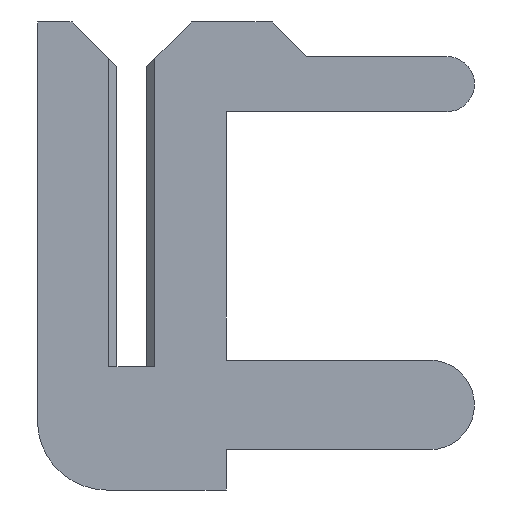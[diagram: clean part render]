
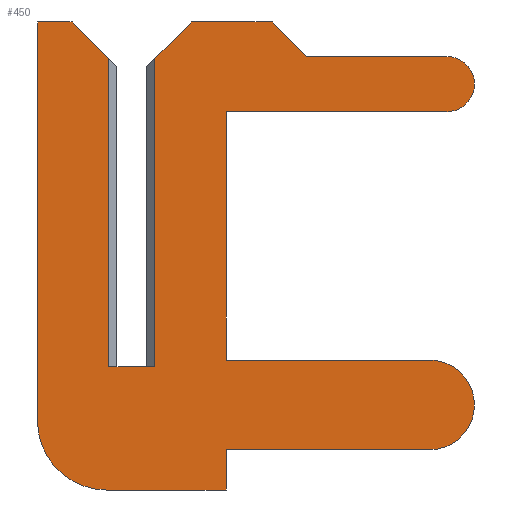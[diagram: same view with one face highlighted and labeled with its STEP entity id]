
A CAD part, left-side view. The second image highlights one B-rep face of the part: STEP entity #450.
In plain terms, the highlighted planar face has unit normal (-1, 0, 0).
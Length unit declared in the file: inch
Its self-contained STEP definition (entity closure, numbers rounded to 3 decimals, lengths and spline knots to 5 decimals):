
#2 = EDGE_CURVE ( 'NONE', #1318, #54, #545, .T. ) ;
#14 = VERTEX_POINT ( 'NONE', #548 ) ;
#23 = DIRECTION ( 'NONE',  ( 0., 0., 1. ) ) ;
#27 = DIRECTION ( 'NONE',  ( 0., -1., 0. ) ) ;
#28 = CARTESIAN_POINT ( 'NONE',  ( -0.01, -0.041, -0.0535 ) ) ;
#37 = ORIENTED_EDGE ( 'NONE', *, *, #387, .F. ) ;
#54 = VERTEX_POINT ( 'NONE', #367 ) ;
#55 = EDGE_CURVE ( 'NONE', #54, #898, #498, .T. ) ;
#56 = CARTESIAN_POINT ( 'NONE',  ( -0.01, 0.01, -0.0235 ) ) ;
#67 = ORIENTED_EDGE ( 'NONE', *, *, #483, .F. ) ;
#74 = EDGE_CURVE ( 'NONE', #751, #1318, #512, .T. ) ;
#81 = CARTESIAN_POINT ( 'NONE',  ( -0.01, -0.041, 0.111 ) ) ;
#88 = EDGE_CURVE ( 'NONE', #524, #998, #677, .T. ) ;
#91 = VECTOR ( 'NONE', #1185, 39.37008 ) ;
#104 = LINE ( 'NONE', #488, #641 ) ;
#136 = VERTEX_POINT ( 'NONE', #81 ) ;
#157 = CARTESIAN_POINT ( 'NONE',  ( -0.01, -0.041, -0.036 ) ) ;
#161 = VECTOR ( 'NONE', #27, 39.37008 ) ;
#166 = DIRECTION ( 'NONE',  ( 0., 0., -1. ) ) ;
#176 = ORIENTED_EDGE ( 'NONE', *, *, #1001, .F. ) ;
#197 = LINE ( 'NONE', #1285, #1102 ) ;
#202 = DIRECTION ( 'NONE',  ( 0., -1., 0. ) ) ;
#209 = CARTESIAN_POINT ( 'NONE',  ( -0.01, -0.01, 0. ) ) ;
#228 = DIRECTION ( 'NONE',  ( 1., 0., 0. ) ) ;
#237 = VERTEX_POINT ( 'NONE', #815 ) ;
#244 = VECTOR ( 'NONE', #202, 39.37008 ) ;
#256 = VERTEX_POINT ( 'NONE', #1148 ) ;
#277 = DIRECTION ( 'NONE',  ( 0., 1., 0. ) ) ;
#278 = CARTESIAN_POINT ( 'NONE',  ( -0.01, -0.061, 0.15 ) ) ;
#291 = EDGE_LOOP ( 'NONE', ( #753, #1279, #332, #1259, #1330, #462, #1212, #788, #603, #879, #866, #913, #1183, #1315, #67, #1342, #808, #37, #176 ) ) ;
#296 = CARTESIAN_POINT ( 'NONE',  ( -0.01, 0.041, 0.15 ) ) ;
#312 = DIRECTION ( 'NONE',  ( 0., -1., 0. ) ) ;
#331 = DIRECTION ( 'NONE',  ( 0., -0.707, 0.707 ) ) ;
#332 = ORIENTED_EDGE ( 'NONE', *, *, #401, .F. ) ;
#340 = DIRECTION ( 'NONE',  ( 0., -0.707, -0.707 ) ) ;
#341 = DIRECTION ( 'NONE',  ( 0., 0., -1. ) ) ;
#350 = EDGE_CURVE ( 'NONE', #535, #14, #661, .T. ) ;
#354 = DIRECTION ( 'NONE',  ( 0., 1., 0. ) ) ;
#358 = VERTEX_POINT ( 'NONE', #1149 ) ;
#367 = CARTESIAN_POINT ( 'NONE',  ( -0.01, -0.1295, -0.036 ) ) ;
#379 = EDGE_CURVE ( 'NONE', #358, #930, #971, .T. ) ;
#387 = EDGE_CURVE ( 'NONE', #931, #734, #726, .T. ) ;
#401 = EDGE_CURVE ( 'NONE', #1282, #1057, #1287, .T. ) ;
#410 = CARTESIAN_POINT ( 'NONE',  ( -0.01, -0.0065, 0.1305 ) ) ;
#412 = DIRECTION ( 'NONE',  ( 1., 0., 0. ) ) ;
#420 = DIRECTION ( 'NONE',  ( -1., 0., 0. ) ) ;
#429 = CARTESIAN_POINT ( 'NONE',  ( -0.01, -0.1295, 0.003 ) ) ;
#446 = CARTESIAN_POINT ( 'NONE',  ( -0.01, 0.011, -0.0235 ) ) ;
#448 = DIRECTION ( 'NONE',  ( 0., 1., 0. ) ) ;
#450 = ADVANCED_FACE ( 'NONE', ( #1218 ), #1050, .T. ) ;
#462 = ORIENTED_EDGE ( 'NONE', *, *, #88, .F. ) ;
#468 = EDGE_CURVE ( 'NONE', #1282, #256, #1239, .T. ) ;
#479 = VECTOR ( 'NONE', #354, 39.37008 ) ;
#483 = EDGE_CURVE ( 'NONE', #930, #136, #197, .T. ) ;
#488 = CARTESIAN_POINT ( 'NONE',  ( -0.01, -0.01, 0.15 ) ) ;
#493 = CARTESIAN_POINT ( 'NONE',  ( -0.01, -0.076, 0.135 ) ) ;
#498 = LINE ( 'NONE', #157, #623 ) ;
#500 = VECTOR ( 'NONE', #1263, 39.37008 ) ;
#512 = LINE ( 'NONE', #1322, #854 ) ;
#513 = LINE ( 'NONE', #410, #1238 ) ;
#517 = EDGE_CURVE ( 'NONE', #136, #751, #825, .T. ) ;
#524 = VERTEX_POINT ( 'NONE', #789 ) ;
#535 = VERTEX_POINT ( 'NONE', #28 ) ;
#540 = EDGE_CURVE ( 'NONE', #898, #535, #973, .T. ) ;
#541 = CARTESIAN_POINT ( 'NONE',  ( -0.01, -0.041, -0.0535 ) ) ;
#542 = DIRECTION ( 'NONE',  ( 1., 0., 0. ) ) ;
#545 = CIRCLE ( 'NONE', #943, 0.0195 ) ;
#548 = CARTESIAN_POINT ( 'NONE',  ( -0.01, 0.011, -0.0535 ) ) ;
#564 = LINE ( 'NONE', #1067, #161 ) ;
#575 = CARTESIAN_POINT ( 'NONE',  ( -0.01, 0.026, 0.15 ) ) ;
#579 = CARTESIAN_POINT ( 'NONE',  ( -0.01, -0.041, 0.003 ) ) ;
#591 = AXIS2_PLACEMENT_3D ( 'NONE', #624, #420, #1312 ) ;
#603 = ORIENTED_EDGE ( 'NONE', *, *, #350, .F. ) ;
#613 = CARTESIAN_POINT ( 'NONE',  ( -0.01, -0.026, 0.15 ) ) ;
#616 = DIRECTION ( 'NONE',  ( 0., 0., 1. ) ) ;
#623 = VECTOR ( 'NONE', #277, 39.37008 ) ;
#624 = CARTESIAN_POINT ( 'NONE',  ( -0.01, 0.011, -0.0235 ) ) ;
#631 = CARTESIAN_POINT ( 'NONE',  ( -0.01, -0.137, 0.123 ) ) ;
#636 = EDGE_CURVE ( 'NONE', #748, #1057, #104, .T. ) ;
#641 = VECTOR ( 'NONE', #166, 39.37008 ) ;
#661 = LINE ( 'NONE', #940, #479 ) ;
#677 = LINE ( 'NONE', #575, #1145 ) ;
#692 = VECTOR ( 'NONE', #312, 39.37008 ) ;
#709 = CARTESIAN_POINT ( 'NONE',  ( -0.01, 0.026, 0.15 ) ) ;
#726 = LINE ( 'NONE', #1253, #1249 ) ;
#734 = VERTEX_POINT ( 'NONE', #493 ) ;
#737 = CARTESIAN_POINT ( 'NONE',  ( -0.01, 0.0065, 0. ) ) ;
#744 = CARTESIAN_POINT ( 'NONE',  ( -0.01, 0.01, 0. ) ) ;
#748 = VERTEX_POINT ( 'NONE', #958 ) ;
#751 = VERTEX_POINT ( 'NONE', #579 ) ;
#753 = ORIENTED_EDGE ( 'NONE', *, *, #1230, .F. ) ;
#761 = CARTESIAN_POINT ( 'NONE',  ( -0.01, -0.041, 0.003 ) ) ;
#765 = CARTESIAN_POINT ( 'NONE',  ( -0.01, 0.0065, 0.1305 ) ) ;
#778 = VECTOR ( 'NONE', #966, 39.37008 ) ;
#788 = ORIENTED_EDGE ( 'NONE', *, *, #1291, .F. ) ;
#789 = CARTESIAN_POINT ( 'NONE',  ( -0.01, 0.041, 0.15 ) ) ;
#793 = CARTESIAN_POINT ( 'NONE',  ( -0.01, 0.041, -0.0235 ) ) ;
#808 = ORIENTED_EDGE ( 'NONE', *, *, #1327, .F. ) ;
#815 = CARTESIAN_POINT ( 'NONE',  ( -0.01, -0.026, 0.15 ) ) ;
#825 = LINE ( 'NONE', #761, #1220 ) ;
#854 = VECTOR ( 'NONE', #1103, 39.37008 ) ;
#866 = ORIENTED_EDGE ( 'NONE', *, *, #55, .F. ) ;
#879 = ORIENTED_EDGE ( 'NONE', *, *, #540, .F. ) ;
#883 = VERTEX_POINT ( 'NONE', #793 ) ;
#885 = AXIS2_PLACEMENT_3D ( 'NONE', #631, #412, #616 ) ;
#886 = LINE ( 'NONE', #765, #1005 ) ;
#896 = DIRECTION ( 'NONE',  ( 0., -1., 0. ) ) ;
#898 = VERTEX_POINT ( 'NONE', #1113 ) ;
#913 = ORIENTED_EDGE ( 'NONE', *, *, #2, .F. ) ;
#927 = DIRECTION ( 'NONE',  ( 0., -0.707, -0.707 ) ) ;
#930 = VERTEX_POINT ( 'NONE', #1127 ) ;
#931 = VERTEX_POINT ( 'NONE', #278 ) ;
#940 = CARTESIAN_POINT ( 'NONE',  ( -0.01, 0.011, -0.0535 ) ) ;
#943 = AXIS2_PLACEMENT_3D ( 'NONE', #982, #542, #23 ) ;
#958 = CARTESIAN_POINT ( 'NONE',  ( -0.01, -0.01, 0.134 ) ) ;
#966 = DIRECTION ( 'NONE',  ( 0., 0., 1. ) ) ;
#971 = CIRCLE ( 'NONE', #885, 0.012 ) ;
#973 = LINE ( 'NONE', #541, #91 ) ;
#982 = CARTESIAN_POINT ( 'NONE',  ( -0.01, -0.1295, -0.0165 ) ) ;
#998 = VERTEX_POINT ( 'NONE', #709 ) ;
#1001 = EDGE_CURVE ( 'NONE', #237, #931, #1146, .T. ) ;
#1005 = VECTOR ( 'NONE', #340, 39.37008 ) ;
#1019 = LINE ( 'NONE', #296, #500 ) ;
#1035 = CIRCLE ( 'NONE', #1241, 0.03 ) ;
#1050 = PLANE ( 'NONE',  #591 ) ;
#1057 = VERTEX_POINT ( 'NONE', #209 ) ;
#1067 = CARTESIAN_POINT ( 'NONE',  ( -0.01, -0.137, 0.135 ) ) ;
#1102 = VECTOR ( 'NONE', #448, 39.37008 ) ;
#1103 = DIRECTION ( 'NONE',  ( 0., -1., 0. ) ) ;
#1113 = CARTESIAN_POINT ( 'NONE',  ( -0.01, -0.041, -0.036 ) ) ;
#1115 = EDGE_CURVE ( 'NONE', #883, #524, #1019, .T. ) ;
#1127 = CARTESIAN_POINT ( 'NONE',  ( -0.01, -0.137, 0.111 ) ) ;
#1145 = VECTOR ( 'NONE', #896, 39.37008 ) ;
#1146 = LINE ( 'NONE', #613, #244 ) ;
#1148 = CARTESIAN_POINT ( 'NONE',  ( -0.01, 0.01, 0.134 ) ) ;
#1149 = CARTESIAN_POINT ( 'NONE',  ( -0.01, -0.137, 0.135 ) ) ;
#1183 = ORIENTED_EDGE ( 'NONE', *, *, #74, .F. ) ;
#1185 = DIRECTION ( 'NONE',  ( 0., 0., -1. ) ) ;
#1212 = ORIENTED_EDGE ( 'NONE', *, *, #1115, .F. ) ;
#1218 = FACE_OUTER_BOUND ( 'NONE', #291, .T. ) ;
#1220 = VECTOR ( 'NONE', #341, 39.37008 ) ;
#1230 = EDGE_CURVE ( 'NONE', #748, #237, #513, .T. ) ;
#1238 = VECTOR ( 'NONE', #331, 39.37008 ) ;
#1239 = LINE ( 'NONE', #56, #778 ) ;
#1241 = AXIS2_PLACEMENT_3D ( 'NONE', #446, #228, #1273 ) ;
#1249 = VECTOR ( 'NONE', #927, 39.37008 ) ;
#1253 = CARTESIAN_POINT ( 'NONE',  ( -0.01, -0.076, 0.135 ) ) ;
#1257 = EDGE_CURVE ( 'NONE', #998, #256, #886, .T. ) ;
#1259 = ORIENTED_EDGE ( 'NONE', *, *, #468, .T. ) ;
#1263 = DIRECTION ( 'NONE',  ( 0., 0., 1. ) ) ;
#1273 = DIRECTION ( 'NONE',  ( 0., 0., 1. ) ) ;
#1279 = ORIENTED_EDGE ( 'NONE', *, *, #636, .T. ) ;
#1282 = VERTEX_POINT ( 'NONE', #744 ) ;
#1285 = CARTESIAN_POINT ( 'NONE',  ( -0.01, -0.041, 0.111 ) ) ;
#1287 = LINE ( 'NONE', #737, #692 ) ;
#1291 = EDGE_CURVE ( 'NONE', #14, #883, #1035, .T. ) ;
#1312 = DIRECTION ( 'NONE',  ( 0., 0., 1. ) ) ;
#1315 = ORIENTED_EDGE ( 'NONE', *, *, #517, .F. ) ;
#1318 = VERTEX_POINT ( 'NONE', #429 ) ;
#1322 = CARTESIAN_POINT ( 'NONE',  ( -0.01, -0.1295, 0.003 ) ) ;
#1327 = EDGE_CURVE ( 'NONE', #734, #358, #564, .T. ) ;
#1330 = ORIENTED_EDGE ( 'NONE', *, *, #1257, .F. ) ;
#1342 = ORIENTED_EDGE ( 'NONE', *, *, #379, .F. ) ;
